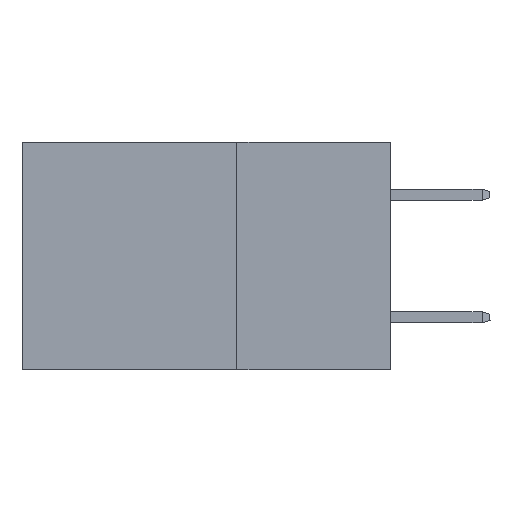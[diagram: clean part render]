
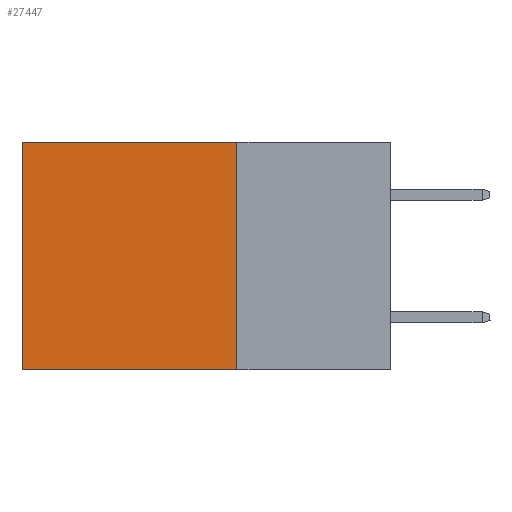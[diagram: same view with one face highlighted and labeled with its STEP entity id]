
A CAD part, left-side view. The second image highlights one B-rep face of the part: STEP entity #27447.
In plain terms, the highlighted planar face has unit normal (-1, 0, 0).
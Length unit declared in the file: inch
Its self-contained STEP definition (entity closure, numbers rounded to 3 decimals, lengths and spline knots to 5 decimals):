
#447 = CARTESIAN_POINT ( 'NONE',  ( 0.2875, 0.6, 0. ) ) ;
#772 = VERTEX_POINT ( 'NONE', #10141 ) ;
#1237 = VERTEX_POINT ( 'NONE', #25357 ) ;
#1636 = DIRECTION ( 'NONE',  ( 1., 0., 0. ) ) ;
#1760 = CARTESIAN_POINT ( 'NONE',  ( 0.2875, 0.25, 0. ) ) ;
#2549 = DIRECTION ( 'NONE',  ( 0., 1., 0. ) ) ;
#3821 = DIRECTION ( 'NONE',  ( 0., 0., -1. ) ) ;
#6050 = EDGE_LOOP ( 'NONE', ( #26641, #7457, #21775, #10186 ) ) ;
#6265 = CARTESIAN_POINT ( 'NONE',  ( 0.2875, 0.6, 0. ) ) ;
#7404 = AXIS2_PLACEMENT_3D ( 'NONE', #32595, #1636, #11724 ) ;
#7457 = ORIENTED_EDGE ( 'NONE', *, *, #32169, .F. ) ;
#7717 = CARTESIAN_POINT ( 'NONE',  ( 0.2875, 0.25, -0.37 ) ) ;
#9999 = EDGE_CURVE ( 'NONE', #18931, #19405, #11374, .T. ) ;
#10141 = CARTESIAN_POINT ( 'NONE',  ( 0.2875, 0.25, -0.37 ) ) ;
#10186 = ORIENTED_EDGE ( 'NONE', *, *, #19804, .T. ) ;
#11237 = DIRECTION ( 'NONE',  ( 0., 1., 0. ) ) ;
#11374 = LINE ( 'NONE', #6265, #31663 ) ;
#11462 = EDGE_CURVE ( 'NONE', #1237, #772, #23786, .T. ) ;
#11724 = DIRECTION ( 'NONE',  ( 0., 0., -1. ) ) ;
#12282 = VECTOR ( 'NONE', #2549, 39.37008 ) ;
#12369 = VECTOR ( 'NONE', #3821, 39.37008 ) ;
#17225 = FACE_OUTER_BOUND ( 'NONE', #6050, .T. ) ;
#18931 = VERTEX_POINT ( 'NONE', #447 ) ;
#19203 = LINE ( 'NONE', #7717, #12282 ) ;
#19215 = VECTOR ( 'NONE', #11237, 39.37008 ) ;
#19405 = VERTEX_POINT ( 'NONE', #20606 ) ;
#19804 = EDGE_CURVE ( 'NONE', #1237, #18931, #32587, .T. ) ;
#20606 = CARTESIAN_POINT ( 'NONE',  ( 0.2875, 0.6, -0.37 ) ) ;
#21155 = CARTESIAN_POINT ( 'NONE',  ( 0.2875, 0.25, 0. ) ) ;
#21775 = ORIENTED_EDGE ( 'NONE', *, *, #11462, .F. ) ;
#22193 = PLANE ( 'NONE',  #7404 ) ;
#23786 = LINE ( 'NONE', #1760, #12369 ) ;
#24438 = DIRECTION ( 'NONE',  ( 0., 0., -1. ) ) ;
#25357 = CARTESIAN_POINT ( 'NONE',  ( 0.2875, 0.25, 0. ) ) ;
#26641 = ORIENTED_EDGE ( 'NONE', *, *, #9999, .T. ) ;
#27447 = ADVANCED_FACE ( 'NONE', ( #17225 ), #22193, .F. ) ;
#31663 = VECTOR ( 'NONE', #24438, 39.37008 ) ;
#32169 = EDGE_CURVE ( 'NONE', #772, #19405, #19203, .T. ) ;
#32587 = LINE ( 'NONE', #21155, #19215 ) ;
#32595 = CARTESIAN_POINT ( 'NONE',  ( 0.2875, 0.25, 0. ) ) ;
